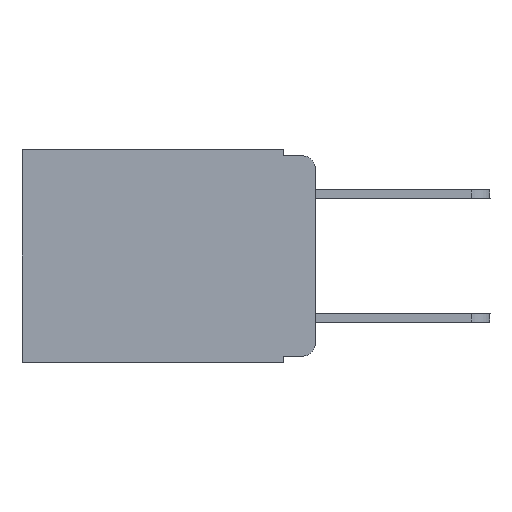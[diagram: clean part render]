
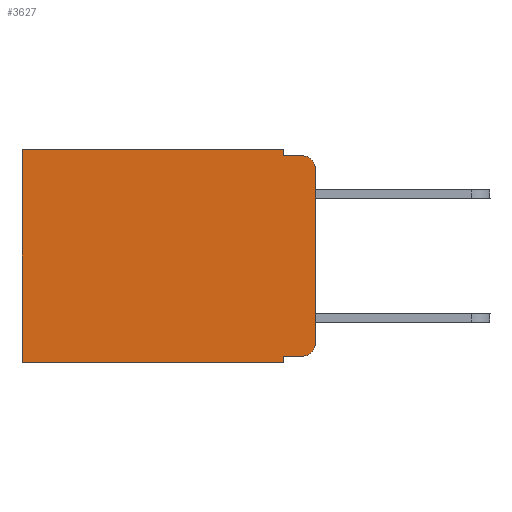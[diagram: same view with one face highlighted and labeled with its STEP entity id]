
A CAD part, left-side view. The second image highlights one B-rep face of the part: STEP entity #3627.
In plain terms, the highlighted planar face has unit normal (-1, 0, 0).
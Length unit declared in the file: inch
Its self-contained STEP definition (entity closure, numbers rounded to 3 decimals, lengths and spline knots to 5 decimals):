
#160 = ORIENTED_EDGE ( 'NONE', *, *, #19783, .F. ) ;
#204 = VERTEX_POINT ( 'NONE', #15041 ) ;
#226 = CARTESIAN_POINT ( 'NONE',  ( 0.298, 0.02, -0.03 ) ) ;
#271 = CARTESIAN_POINT ( 'NONE',  ( 0.298, 0.051, -0.01 ) ) ;
#696 = FACE_OUTER_BOUND ( 'NONE', #19192, .T. ) ;
#729 = CARTESIAN_POINT ( 'NONE',  ( 0.298, 0.02, -0.333 ) ) ;
#808 = ORIENTED_EDGE ( 'NONE', *, *, #4063, .T. ) ;
#958 = CARTESIAN_POINT ( 'NONE',  ( 0.298, 0.051, 0. ) ) ;
#1124 = CARTESIAN_POINT ( 'NONE',  ( 0.298, 0.051, 0. ) ) ;
#1347 = LINE ( 'NONE', #15093, #1482 ) ;
#1482 = VECTOR ( 'NONE', #11580, 39.37008 ) ;
#1928 = DIRECTION ( 'NONE',  ( 0., 0., -1. ) ) ;
#2003 = LINE ( 'NONE', #3646, #10748 ) ;
#2495 = VECTOR ( 'NONE', #15404, 39.37008 ) ;
#2502 = EDGE_CURVE ( 'NONE', #9467, #3601, #12103, .T. ) ;
#2533 = DIRECTION ( 'NONE',  ( 0., 0., -1. ) ) ;
#2724 = DIRECTION ( 'NONE',  ( 0., -1., 0. ) ) ;
#3601 = VERTEX_POINT ( 'NONE', #17756 ) ;
#3627 = ADVANCED_FACE ( 'NONE', ( #696 ), #21264, .F. ) ;
#3646 = CARTESIAN_POINT ( 'NONE',  ( 0.298, 0.473, 0. ) ) ;
#3842 = EDGE_CURVE ( 'NONE', #9872, #17331, #1347, .T. ) ;
#3863 = CARTESIAN_POINT ( 'NONE',  ( 0.298, 0., -0.03 ) ) ;
#4063 = EDGE_CURVE ( 'NONE', #17331, #204, #14484, .T. ) ;
#4078 = CARTESIAN_POINT ( 'NONE',  ( 0.298, 0.02, -0.313 ) ) ;
#4542 = DIRECTION ( 'NONE',  ( 0., 0., -1. ) ) ;
#5176 = CARTESIAN_POINT ( 'NONE',  ( 0.298, 0.051, -0.343 ) ) ;
#5737 = DIRECTION ( 'NONE',  ( 0., 0., -1. ) ) ;
#5911 = VECTOR ( 'NONE', #7514, 39.37008 ) ;
#6107 = ORIENTED_EDGE ( 'NONE', *, *, #12256, .F. ) ;
#6253 = ORIENTED_EDGE ( 'NONE', *, *, #2502, .T. ) ;
#6805 = LINE ( 'NONE', #10423, #18873 ) ;
#6919 = DIRECTION ( 'NONE',  ( 0., 1., 0. ) ) ;
#7259 = EDGE_CURVE ( 'NONE', #9849, #17691, #20487, .T. ) ;
#7514 = DIRECTION ( 'NONE',  ( 0., 0., -1. ) ) ;
#7600 = DIRECTION ( 'NONE',  ( -1., 0., 0. ) ) ;
#8582 = CARTESIAN_POINT ( 'NONE',  ( 0.298, 0., 0. ) ) ;
#8924 = CARTESIAN_POINT ( 'NONE',  ( 0.298, 0.051, -0.333 ) ) ;
#9077 = CARTESIAN_POINT ( 'NONE',  ( 0.298, 0., 0. ) ) ;
#9467 = VERTEX_POINT ( 'NONE', #958 ) ;
#9849 = VERTEX_POINT ( 'NONE', #3863 ) ;
#9872 = VERTEX_POINT ( 'NONE', #8924 ) ;
#10423 = CARTESIAN_POINT ( 'NONE',  ( 0.298, 0., -0.343 ) ) ;
#10748 = VECTOR ( 'NONE', #18518, 39.37008 ) ;
#10864 = CARTESIAN_POINT ( 'NONE',  ( 0.298, 0.051, -0.01 ) ) ;
#11135 = VECTOR ( 'NONE', #2724, 39.37008 ) ;
#11144 = CARTESIAN_POINT ( 'NONE',  ( 0.298, 0., 0. ) ) ;
#11149 = CARTESIAN_POINT ( 'NONE',  ( 0.298, 0.473, -0.343 ) ) ;
#11432 = EDGE_CURVE ( 'NONE', #9872, #14500, #16210, .T. ) ;
#11580 = DIRECTION ( 'NONE',  ( 0., -1., 0. ) ) ;
#12103 = LINE ( 'NONE', #8582, #2495 ) ;
#12161 = LINE ( 'NONE', #9077, #20869 ) ;
#12256 = EDGE_CURVE ( 'NONE', #9849, #204, #12161, .T. ) ;
#12564 = ORIENTED_EDGE ( 'NONE', *, *, #7259, .T. ) ;
#12587 = DIRECTION ( 'NONE',  ( 1., 0., 0. ) ) ;
#13861 = VECTOR ( 'NONE', #5737, 39.37008 ) ;
#14029 = ORIENTED_EDGE ( 'NONE', *, *, #17605, .T. ) ;
#14104 = CARTESIAN_POINT ( 'NONE',  ( 0.298, 0.051, 0. ) ) ;
#14484 = CIRCLE ( 'NONE', #17299, 0.02 ) ;
#14500 = VERTEX_POINT ( 'NONE', #5176 ) ;
#14814 = AXIS2_PLACEMENT_3D ( 'NONE', #11144, #12587, #4542 ) ;
#14953 = EDGE_CURVE ( 'NONE', #14500, #16200, #6805, .T. ) ;
#15029 = EDGE_CURVE ( 'NONE', #19130, #17691, #17805, .T. ) ;
#15041 = CARTESIAN_POINT ( 'NONE',  ( 0.298, 0., -0.313 ) ) ;
#15093 = CARTESIAN_POINT ( 'NONE',  ( 0.298, 0.051, -0.333 ) ) ;
#15404 = DIRECTION ( 'NONE',  ( 0., 1., 0. ) ) ;
#16200 = VERTEX_POINT ( 'NONE', #11149 ) ;
#16210 = LINE ( 'NONE', #1124, #13861 ) ;
#16515 = ORIENTED_EDGE ( 'NONE', *, *, #15029, .F. ) ;
#16953 = DIRECTION ( 'NONE',  ( 0., 0., -1. ) ) ;
#17063 = DIRECTION ( 'NONE',  ( -1., 0., 0. ) ) ;
#17299 = AXIS2_PLACEMENT_3D ( 'NONE', #4078, #7600, #2533 ) ;
#17331 = VERTEX_POINT ( 'NONE', #729 ) ;
#17408 = CARTESIAN_POINT ( 'NONE',  ( 0.298, 0.02, -0.01 ) ) ;
#17605 = EDGE_CURVE ( 'NONE', #3601, #16200, #2003, .T. ) ;
#17688 = AXIS2_PLACEMENT_3D ( 'NONE', #226, #17063, #16953 ) ;
#17691 = VERTEX_POINT ( 'NONE', #17408 ) ;
#17756 = CARTESIAN_POINT ( 'NONE',  ( 0.298, 0.473, 0. ) ) ;
#17805 = LINE ( 'NONE', #10864, #11135 ) ;
#18518 = DIRECTION ( 'NONE',  ( 0., 0., -1. ) ) ;
#18736 = ORIENTED_EDGE ( 'NONE', *, *, #11432, .F. ) ;
#18873 = VECTOR ( 'NONE', #6919, 39.37008 ) ;
#19130 = VERTEX_POINT ( 'NONE', #271 ) ;
#19189 = LINE ( 'NONE', #14104, #5911 ) ;
#19192 = EDGE_LOOP ( 'NONE', ( #6107, #12564, #16515, #160, #6253, #14029, #19347, #18736, #20850, #808 ) ) ;
#19347 = ORIENTED_EDGE ( 'NONE', *, *, #14953, .F. ) ;
#19783 = EDGE_CURVE ( 'NONE', #9467, #19130, #19189, .T. ) ;
#20487 = CIRCLE ( 'NONE', #17688, 0.02 ) ;
#20850 = ORIENTED_EDGE ( 'NONE', *, *, #3842, .T. ) ;
#20869 = VECTOR ( 'NONE', #1928, 39.37008 ) ;
#21264 = PLANE ( 'NONE',  #14814 ) ;
